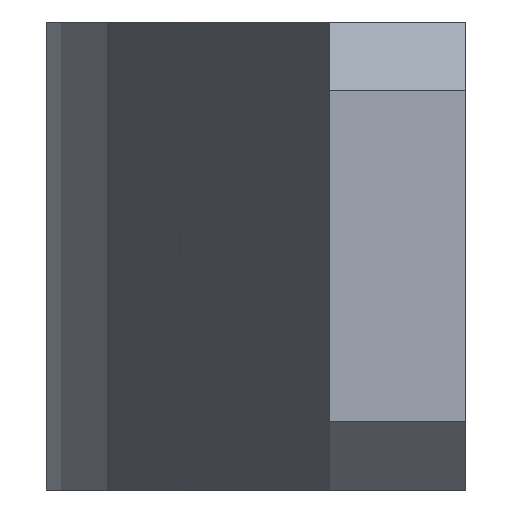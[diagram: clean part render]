
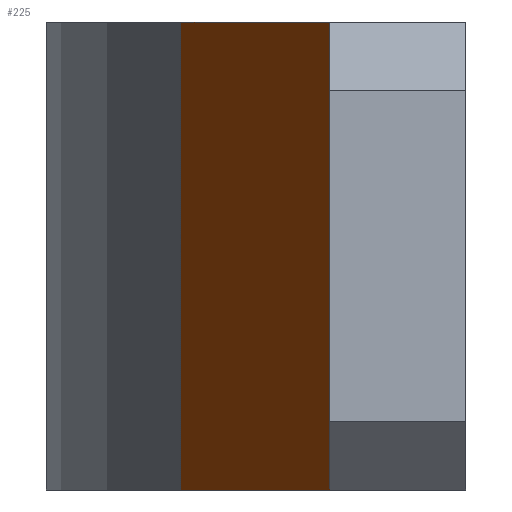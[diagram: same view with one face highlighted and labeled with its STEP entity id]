
A CAD part, left-side view. The second image highlights one B-rep face of the part: STEP entity #225.
In plain terms, the highlighted planar face has unit normal (-0.459, 0.888, 0).
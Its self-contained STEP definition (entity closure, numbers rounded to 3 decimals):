
#2 = VERTEX_POINT ( 'NONE', #416 ) ;
#12 = CARTESIAN_POINT ( 'NONE',  ( -12.932, 3.472, 45.967 ) ) ;
#29 = ORIENTED_EDGE ( 'NONE', *, *, #144, .T. ) ;
#44 = DIRECTION ( 'NONE',  ( -0.888, -0.459, 0. ) ) ;
#57 = VECTOR ( 'NONE', #88, 1000. ) ;
#65 = EDGE_CURVE ( 'NONE', #470, #2, #639, .T. ) ;
#88 = DIRECTION ( 'NONE',  ( 0., 0., -1. ) ) ;
#98 = DIRECTION ( 'NONE',  ( 0., 0., 1. ) ) ;
#114 = CARTESIAN_POINT ( 'NONE',  ( -4.14, 8.014, 5.461 ) ) ;
#144 = EDGE_CURVE ( 'NONE', #180, #470, #419, .T. ) ;
#155 = CARTESIAN_POINT ( 'NONE',  ( -19.653, 0., -5.461 ) ) ;
#162 = DIRECTION ( 'NONE',  ( -0.459, 0.888, 0. ) ) ;
#180 = VERTEX_POINT ( 'NONE', #598 ) ;
#222 = VERTEX_POINT ( 'NONE', #683 ) ;
#225 = ADVANCED_FACE ( 'NONE', ( #360 ), #516, .T. ) ;
#251 = VECTOR ( 'NONE', #98, 1000. ) ;
#277 = DIRECTION ( 'NONE',  ( 0.888, 0.459, 0. ) ) ;
#284 = DIRECTION ( 'NONE',  ( -0.888, -0.459, 0. ) ) ;
#289 = CARTESIAN_POINT ( 'NONE',  ( -4.14, 8.014, 45.967 ) ) ;
#292 = LINE ( 'NONE', #315, #588 ) ;
#315 = CARTESIAN_POINT ( 'NONE',  ( -4.14, 8.014, -5.461 ) ) ;
#328 = EDGE_LOOP ( 'NONE', ( #29, #664, #527, #489 ) ) ;
#332 = VECTOR ( 'NONE', #277, 1000. ) ;
#360 = FACE_OUTER_BOUND ( 'NONE', #328, .T. ) ;
#369 = LINE ( 'NONE', #12, #57 ) ;
#416 = CARTESIAN_POINT ( 'NONE',  ( -12.932, 3.472, 5.461 ) ) ;
#419 = LINE ( 'NONE', #155, #251 ) ;
#454 = CARTESIAN_POINT ( 'NONE',  ( -19.653, 0., 5.461 ) ) ;
#470 = VERTEX_POINT ( 'NONE', #454 ) ;
#476 = AXIS2_PLACEMENT_3D ( 'NONE', #289, #162, #44 ) ;
#489 = ORIENTED_EDGE ( 'NONE', *, *, #532, .T. ) ;
#516 = PLANE ( 'NONE',  #476 ) ;
#527 = ORIENTED_EDGE ( 'NONE', *, *, #593, .T. ) ;
#532 = EDGE_CURVE ( 'NONE', #222, #180, #292, .T. ) ;
#588 = VECTOR ( 'NONE', #284, 1000. ) ;
#593 = EDGE_CURVE ( 'NONE', #2, #222, #369, .T. ) ;
#598 = CARTESIAN_POINT ( 'NONE',  ( -19.653, 0., -5.461 ) ) ;
#639 = LINE ( 'NONE', #114, #332 ) ;
#664 = ORIENTED_EDGE ( 'NONE', *, *, #65, .T. ) ;
#683 = CARTESIAN_POINT ( 'NONE',  ( -12.932, 3.472, -5.461 ) ) ;
